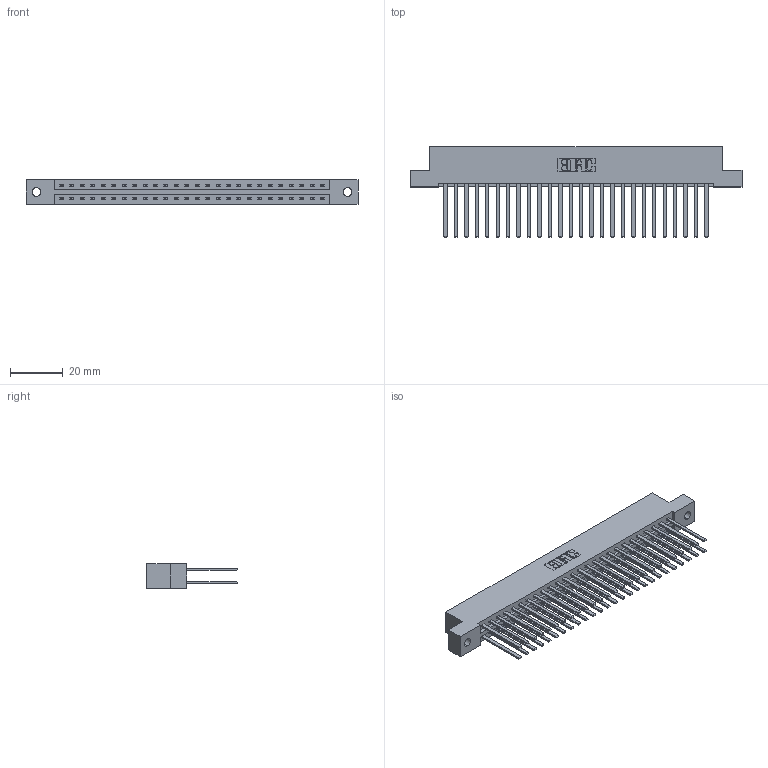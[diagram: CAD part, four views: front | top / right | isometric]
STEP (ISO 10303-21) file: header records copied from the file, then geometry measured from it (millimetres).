
FILE_DESCRIPTION (( 'STEP AP203' ), '1' );
FILE_NAME ('387-052-544-202.STEP', '2019-10-19T03:32:14', ( '' ), ( '' ), 'SwSTEP 2.0', 'SolidWorks 2016', '' );
FILE_SCHEMA (( 'CONFIG_CONTROL_DESIGN' ));
Length unit declared in the file: inch
Products named in the file (3): 387-052-544-202; 345-292-001_345-293-144; 337 Part_Flush Mounting Lugs - 0.128 Dia
Assembly tree (53 placements, depth 2):
  387-052-544-202
    337 Part_Flush Mounting Lugs - 0.128 Dia
    345-292-001_345-293-144  x52
Bounding box: 126.03 x 34.3 x 9.4 mm (x, y, z)
Volume: 13761.8 mm3; surface area: 17510.9 mm2
Topology: 53 solids, 53 shells, 2610 faces, 7747 edges, 5094 vertices
Faces by surface type: plane 1838, cylinder 772
Entity records: 22047 total; most frequent: CARTESIAN_POINT 3726, ORIENTED_EDGE 3662, DIRECTION 3195, EDGE_CURVE 1831, VECTOR 1707, LINE 1707, VERTEX_POINT 1218, AXIS2_PLACEMENT_3D 744
